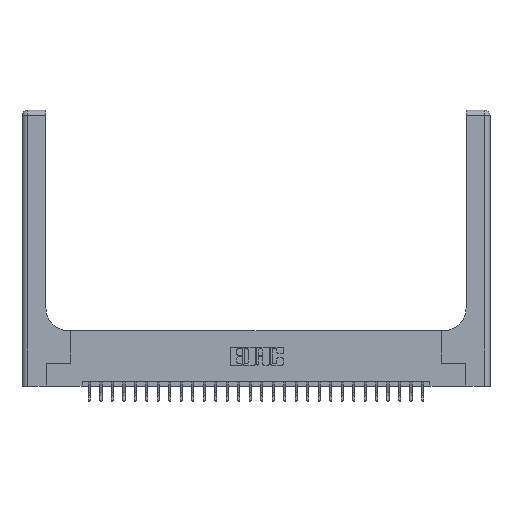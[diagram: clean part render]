
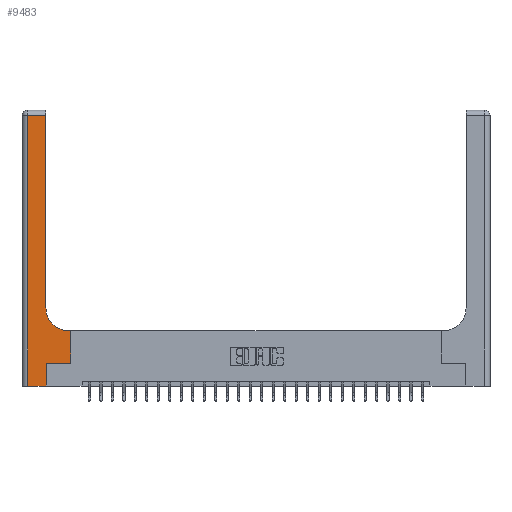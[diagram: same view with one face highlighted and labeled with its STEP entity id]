
A CAD part, top view. The second image highlights one B-rep face of the part: STEP entity #9483.
In plain terms, the highlighted planar face has unit normal (0, 0, 1).
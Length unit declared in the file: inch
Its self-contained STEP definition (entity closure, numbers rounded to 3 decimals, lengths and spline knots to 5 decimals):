
#368 = DIRECTION ( 'NONE',  ( -1., 0., 0. ) ) ;
#548 = EDGE_CURVE ( 'NONE', #19884, #2157, #17198, .T. ) ;
#2082 = VERTEX_POINT ( 'NONE', #21535 ) ;
#2157 = VERTEX_POINT ( 'NONE', #7484 ) ;
#4618 = CIRCLE ( 'NONE', #18971, 0.25 ) ;
#5351 = ORIENTED_EDGE ( 'NONE', *, *, #11614, .T. ) ;
#5506 = CARTESIAN_POINT ( 'NONE',  ( 0.51, 0.6, 0.37 ) ) ;
#5616 = LINE ( 'NONE', #25604, #25470 ) ;
#6470 = EDGE_CURVE ( 'NONE', #20222, #26036, #18564, .T. ) ;
#6720 = CARTESIAN_POINT ( 'NONE',  ( 0.265, 0.25, 0.37 ) ) ;
#6991 = VECTOR ( 'NONE', #10397, 39.37008 ) ;
#7093 = CARTESIAN_POINT ( 'NONE',  ( 0., 0., 0.37 ) ) ;
#7484 = CARTESIAN_POINT ( 'NONE',  ( 0.528, 0.25, 0.37 ) ) ;
#8362 = ORIENTED_EDGE ( 'NONE', *, *, #17549, .T. ) ;
#9424 = LINE ( 'NONE', #7093, #19854 ) ;
#9483 = ADVANCED_FACE ( 'NONE', ( #22424 ), #24628, .F. ) ;
#9591 = DIRECTION ( 'NONE',  ( -1., 0., 0. ) ) ;
#10103 = ORIENTED_EDGE ( 'NONE', *, *, #6470, .T. ) ;
#10397 = DIRECTION ( 'NONE',  ( 0., 1., 0. ) ) ;
#10607 = VECTOR ( 'NONE', #22194, 39.37008 ) ;
#10653 = CARTESIAN_POINT ( 'NONE',  ( 0.06, 2.94, 0.37 ) ) ;
#10691 = CARTESIAN_POINT ( 'NONE',  ( 0.26, 2.94, 0.37 ) ) ;
#10799 = CARTESIAN_POINT ( 'NONE',  ( 0.26, 0.6, 0.37 ) ) ;
#10800 = EDGE_CURVE ( 'NONE', #23579, #19884, #24264, .T. ) ;
#11026 = DIRECTION ( 'NONE',  ( 0., 0., -1. ) ) ;
#11185 = EDGE_CURVE ( 'NONE', #26036, #23586, #5616, .T. ) ;
#11445 = EDGE_CURVE ( 'NONE', #20783, #20222, #4618, .T. ) ;
#11451 = AXIS2_PLACEMENT_3D ( 'NONE', #14460, #12309, #25021 ) ;
#11614 = EDGE_CURVE ( 'NONE', #2082, #23579, #9424, .T. ) ;
#12309 = DIRECTION ( 'NONE',  ( 0., 0., -1. ) ) ;
#12420 = CARTESIAN_POINT ( 'NONE',  ( 0.26, 3., 0.37 ) ) ;
#12913 = CARTESIAN_POINT ( 'NONE',  ( 0.26, 0.85, 0.37 ) ) ;
#13829 = CARTESIAN_POINT ( 'NONE',  ( 0.265, 0., 0.37 ) ) ;
#14059 = EDGE_LOOP ( 'NONE', ( #10103, #16083, #8362, #5351, #20571, #21147, #18195, #23136, #25522 ) ) ;
#14460 = CARTESIAN_POINT ( 'NONE',  ( 0., 3., 0.37 ) ) ;
#15003 = DIRECTION ( 'NONE',  ( 1., 0., 0. ) ) ;
#15361 = VECTOR ( 'NONE', #22611, 39.37008 ) ;
#15657 = DIRECTION ( 'NONE',  ( 1., 0., 0. ) ) ;
#15806 = CARTESIAN_POINT ( 'NONE',  ( 0.265, 0.25, 0.37 ) ) ;
#16083 = ORIENTED_EDGE ( 'NONE', *, *, #11185, .T. ) ;
#16589 = CARTESIAN_POINT ( 'NONE',  ( 0.06, 3., 0.37 ) ) ;
#16904 = CARTESIAN_POINT ( 'NONE',  ( 0.265, 0., 0.37 ) ) ;
#17039 = CARTESIAN_POINT ( 'NONE',  ( 0.51, 0.85, 0.37 ) ) ;
#17198 = LINE ( 'NONE', #6720, #19370 ) ;
#17549 = EDGE_CURVE ( 'NONE', #23586, #2082, #20411, .T. ) ;
#18195 = ORIENTED_EDGE ( 'NONE', *, *, #21529, .T. ) ;
#18504 = VECTOR ( 'NONE', #22147, 39.37008 ) ;
#18564 = LINE ( 'NONE', #12420, #6991 ) ;
#18971 = AXIS2_PLACEMENT_3D ( 'NONE', #17039, #11026, #19090 ) ;
#19090 = DIRECTION ( 'NONE',  ( 1., 0., 0. ) ) ;
#19110 = LINE ( 'NONE', #10799, #20294 ) ;
#19370 = VECTOR ( 'NONE', #15003, 39.37008 ) ;
#19854 = VECTOR ( 'NONE', #15657, 39.37008 ) ;
#19884 = VERTEX_POINT ( 'NONE', #15806 ) ;
#20222 = VERTEX_POINT ( 'NONE', #12913 ) ;
#20294 = VECTOR ( 'NONE', #368, 39.37008 ) ;
#20411 = LINE ( 'NONE', #16589, #15361 ) ;
#20536 = VERTEX_POINT ( 'NONE', #22722 ) ;
#20571 = ORIENTED_EDGE ( 'NONE', *, *, #10800, .T. ) ;
#20783 = VERTEX_POINT ( 'NONE', #5506 ) ;
#21024 = EDGE_CURVE ( 'NONE', #20536, #20783, #19110, .T. ) ;
#21147 = ORIENTED_EDGE ( 'NONE', *, *, #548, .T. ) ;
#21529 = EDGE_CURVE ( 'NONE', #2157, #20536, #26128, .T. ) ;
#21535 = CARTESIAN_POINT ( 'NONE',  ( 0.06, 0., 0.37 ) ) ;
#22147 = DIRECTION ( 'NONE',  ( 0., 1., 0. ) ) ;
#22194 = DIRECTION ( 'NONE',  ( 0., 1., 0. ) ) ;
#22424 = FACE_OUTER_BOUND ( 'NONE', #14059, .T. ) ;
#22611 = DIRECTION ( 'NONE',  ( 0., -1., 0. ) ) ;
#22722 = CARTESIAN_POINT ( 'NONE',  ( 0.528, 0.6, 0.37 ) ) ;
#23136 = ORIENTED_EDGE ( 'NONE', *, *, #21024, .T. ) ;
#23579 = VERTEX_POINT ( 'NONE', #16904 ) ;
#23586 = VERTEX_POINT ( 'NONE', #10653 ) ;
#24264 = LINE ( 'NONE', #13829, #10607 ) ;
#24628 = PLANE ( 'NONE',  #11451 ) ;
#25021 = DIRECTION ( 'NONE',  ( -1., 0., 0. ) ) ;
#25470 = VECTOR ( 'NONE', #9591, 39.37008 ) ;
#25522 = ORIENTED_EDGE ( 'NONE', *, *, #11445, .T. ) ;
#25604 = CARTESIAN_POINT ( 'NONE',  ( 0., 2.94, 0.37 ) ) ;
#26036 = VERTEX_POINT ( 'NONE', #10691 ) ;
#26128 = LINE ( 'NONE', #26550, #18504 ) ;
#26550 = CARTESIAN_POINT ( 'NONE',  ( 0.528, 0.25, 0.37 ) ) ;
